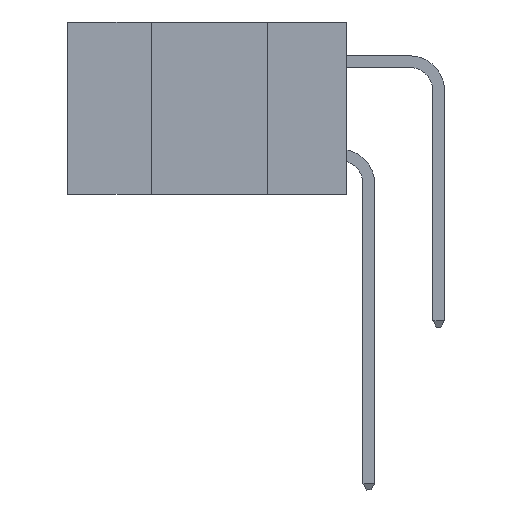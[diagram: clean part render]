
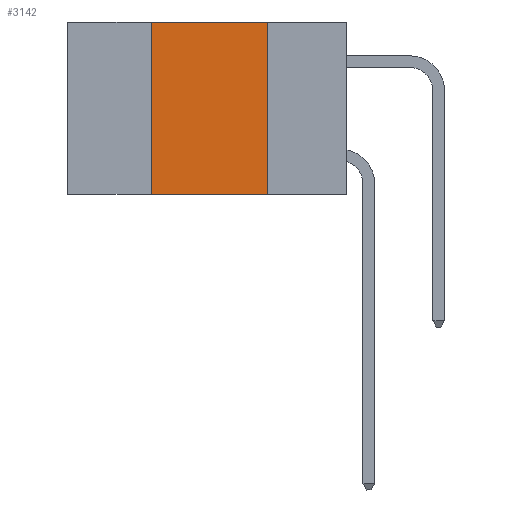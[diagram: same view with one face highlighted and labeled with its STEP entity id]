
A CAD part, left-side view. The second image highlights one B-rep face of the part: STEP entity #3142.
In plain terms, the highlighted planar face has unit normal (-1, 0, 0).
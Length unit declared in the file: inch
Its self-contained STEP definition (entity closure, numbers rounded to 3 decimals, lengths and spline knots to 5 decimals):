
#132 = EDGE_CURVE ( 'NONE', #9930, #8604, #9926, .T. ) ;
#733 = EDGE_LOOP ( 'NONE', ( #5059, #9522, #7864, #9994 ) ) ;
#983 = VECTOR ( 'NONE', #3069, 39.37008 ) ;
#984 = DIRECTION ( 'NONE',  ( 0., 0., -1. ) ) ;
#1002 = LINE ( 'NONE', #7367, #3867 ) ;
#1086 = DIRECTION ( 'NONE',  ( 0., 0., 1. ) ) ;
#1973 = EDGE_CURVE ( 'NONE', #8812, #3475, #8154, .T. ) ;
#2065 = CARTESIAN_POINT ( 'NONE',  ( 0., 0.17, 0. ) ) ;
#2411 = DIRECTION ( 'NONE',  ( 0., -1., 0. ) ) ;
#3069 = DIRECTION ( 'NONE',  ( 0., 0., -1. ) ) ;
#3142 = ADVANCED_FACE ( 'NONE', ( #7765 ), #7303, .F. ) ;
#3166 = CARTESIAN_POINT ( 'NONE',  ( 0., 0.17, -0.37 ) ) ;
#3181 = VECTOR ( 'NONE', #1086, 39.37008 ) ;
#3328 = CARTESIAN_POINT ( 'NONE',  ( 0., 0.42, 0. ) ) ;
#3475 = VERTEX_POINT ( 'NONE', #3166 ) ;
#3560 = EDGE_CURVE ( 'NONE', #8604, #8812, #9092, .T. ) ;
#3637 = CARTESIAN_POINT ( 'NONE',  ( 0., 0.6, 0. ) ) ;
#3797 = CARTESIAN_POINT ( 'NONE',  ( 0., 0.17, 0. ) ) ;
#3867 = VECTOR ( 'NONE', #5626, 39.37008 ) ;
#5059 = ORIENTED_EDGE ( 'NONE', *, *, #1973, .F. ) ;
#5626 = DIRECTION ( 'NONE',  ( 0., -1., 0. ) ) ;
#7303 = PLANE ( 'NONE',  #8930 ) ;
#7367 = CARTESIAN_POINT ( 'NONE',  ( 0., 0.6, -0.37 ) ) ;
#7765 = FACE_OUTER_BOUND ( 'NONE', #733, .T. ) ;
#7864 = ORIENTED_EDGE ( 'NONE', *, *, #132, .F. ) ;
#8154 = LINE ( 'NONE', #2065, #983 ) ;
#8255 = CARTESIAN_POINT ( 'NONE',  ( 0., 0.42, 0. ) ) ;
#8396 = EDGE_CURVE ( 'NONE', #9930, #3475, #1002, .T. ) ;
#8604 = VERTEX_POINT ( 'NONE', #3328 ) ;
#8627 = DIRECTION ( 'NONE',  ( 1., 0., 0. ) ) ;
#8812 = VERTEX_POINT ( 'NONE', #3797 ) ;
#8930 = AXIS2_PLACEMENT_3D ( 'NONE', #9219, #8627, #984 ) ;
#9092 = LINE ( 'NONE', #3637, #9329 ) ;
#9219 = CARTESIAN_POINT ( 'NONE',  ( 0., 0.6, 0. ) ) ;
#9329 = VECTOR ( 'NONE', #2411, 39.37008 ) ;
#9522 = ORIENTED_EDGE ( 'NONE', *, *, #3560, .F. ) ;
#9926 = LINE ( 'NONE', #8255, #3181 ) ;
#9930 = VERTEX_POINT ( 'NONE', #10915 ) ;
#9994 = ORIENTED_EDGE ( 'NONE', *, *, #8396, .T. ) ;
#10915 = CARTESIAN_POINT ( 'NONE',  ( 0., 0.42, -0.37 ) ) ;
